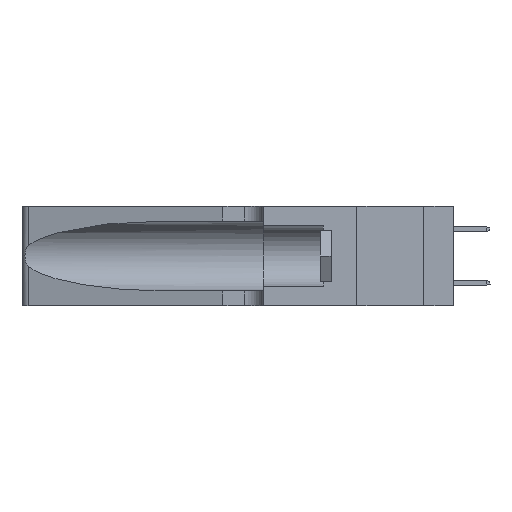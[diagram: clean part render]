
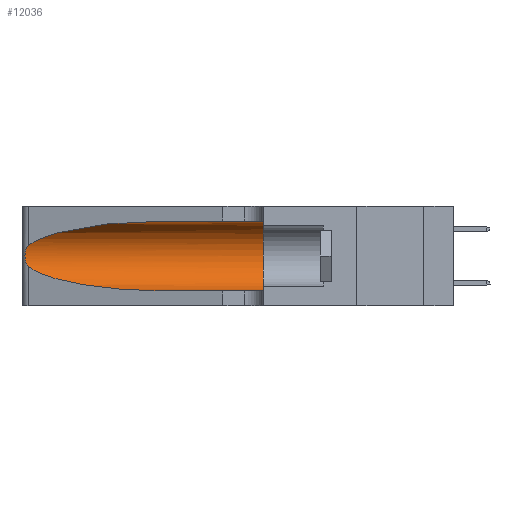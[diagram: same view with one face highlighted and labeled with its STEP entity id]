
A CAD part, left-side view. The second image highlights one B-rep face of the part: STEP entity #12036.
In plain terms, the highlighted cylindrical face has radius 3.308 mm (diameter 6.617 mm), a partial arc.
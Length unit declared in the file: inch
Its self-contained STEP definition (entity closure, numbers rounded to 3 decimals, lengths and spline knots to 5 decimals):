
#126 = CARTESIAN_POINT ( 'NONE',  ( 0.1305, 0.72297, 0.31525 ) ) ;
#168 = EDGE_CURVE ( 'NONE', #28024, #10101, #373, .T. ) ;
#373 = LINE ( 'NONE', #2477, #8485 ) ;
#961 = CARTESIAN_POINT ( 'NONE',  ( 0.1305, 0.72297, 0.31525 ) ) ;
#2454 = CARTESIAN_POINT ( 'NONE',  ( 0.1305, 0.35, 0.31525 ) ) ;
#2477 = CARTESIAN_POINT ( 'NONE',  ( 0.1305, 1.61858, 0.31525 ) ) ;
#3458 = EDGE_CURVE ( 'NONE', #17336, #17997, #14928, .T. ) ;
#3808 = CARTESIAN_POINT ( 'NONE',  ( 0.25856, 1.23593, 0.16098 ) ) ;
#3963 = CARTESIAN_POINT ( 'NONE',  ( 0.25789, 1.23486, 0.15765 ) ) ;
#4413 = LINE ( 'NONE', #13510, #17447 ) ;
#4511 = CARTESIAN_POINT ( 'NONE',  ( 0.1305, 0.72297, 0.05475 ) ) ;
#4795 = EDGE_CURVE ( 'NONE', #27685, #5377, #4413, .T. ) ;
#5363 = CARTESIAN_POINT ( 'NONE',  ( 0.2373, 1.15595, 0.08982 ) ) ;
#5377 = VERTEX_POINT ( 'NONE', #28081 ) ;
#7649 = AXIS2_PLACEMENT_3D ( 'NONE', #28971, #24512, #13146 ) ;
#8152 = AXIS2_PLACEMENT_3D ( 'NONE', #21940, #28342, #19832 ) ;
#8485 = VECTOR ( 'NONE', #12420, 39.37008 ) ;
#10094 = CARTESIAN_POINT ( 'NONE',  ( 0.18966, 0.96281, 0.31525 ) ) ;
#10101 = VERTEX_POINT ( 'NONE', #2454 ) ;
#10274 = CARTESIAN_POINT ( 'NONE',  ( 0.25487, 1.22718, 0.14631 ) ) ;
#10445 = CYLINDRICAL_SURFACE ( 'NONE', #8152, 0.13025 ) ;
#10976 = CARTESIAN_POINT ( 'NONE',  ( 0.25854, 1.2359, 0.20912 ) ) ;
#11126 = CARTESIAN_POINT ( 'NONE',  ( 0.25555, 1.22994, 0.2215 ) ) ;
#11644 = EDGE_CURVE ( 'NONE', #10101, #5377, #20506, .T. ) ;
#12036 = ADVANCED_FACE ( 'NONE', ( #12517 ), #10445, .F. ) ;
#12420 = DIRECTION ( 'NONE',  ( 0., -1., 0. ) ) ;
#12517 = FACE_OUTER_BOUND ( 'NONE', #25719, .T. ) ;
#12912 = CARTESIAN_POINT ( 'NONE',  ( 0.25555, 1.22993, 0.14849 ) ) ;
#13146 = DIRECTION ( 'NONE',  ( 0., 0., 1. ) ) ;
#13510 = CARTESIAN_POINT ( 'NONE',  ( 0.1305, 1.61858, 0.05475 ) ) ;
#13924 = ORIENTED_EDGE ( 'NONE', *, *, #28199, .T. ) ;
#14928 = B_SPLINE_CURVE_WITH_KNOTS ( 'NONE', 3,
 ( #19634, #11126, #27082, #26797, #10976, #26934, #26640, #20226, #24425, #3808, #3963, #19775, #12912, #29319 ),
 .UNSPECIFIED., .F., .F.,
 ( 4, 2, 2, 2, 2, 2, 4 ),
 ( 0., 0.00027, 0.00053, 0.00107, 0.0016, 0.00187, 0.00214 ),
 .UNSPECIFIED. ) ;
#16085 = ORIENTED_EDGE ( 'NONE', *, *, #168, .F. ) ;
#16308 = ORIENTED_EDGE ( 'NONE', *, *, #4795, .T. ) ;
#16701 = CARTESIAN_POINT ( 'NONE',  ( 0.1305, 0.72297, 0.05475 ) ) ;
#16946 = CARTESIAN_POINT ( 'NONE',  ( 0.2373, 1.15595, 0.28018 ) ) ;
#17028 =( BOUNDED_CURVE ( )  B_SPLINE_CURVE ( 3, ( #961, #10094, #16946, #21593 ),
 .UNSPECIFIED., .F., .T. ) 
 B_SPLINE_CURVE_WITH_KNOTS ( ( 4, 4 ),
 ( 1.5708, 2.84003 ),
 .UNSPECIFIED. ) 
 CURVE ( )  GEOMETRIC_REPRESENTATION_ITEM ( )  RATIONAL_B_SPLINE_CURVE ( ( 1., 0.87, 0.87, 1. ) ) 
 REPRESENTATION_ITEM ( '' )  );
#17336 = VERTEX_POINT ( 'NONE', #27878 ) ;
#17382 = CARTESIAN_POINT ( 'NONE',  ( 0.25487, 1.22718, 0.14631 ) ) ;
#17447 = VECTOR ( 'NONE', #20089, 39.37008 ) ;
#17997 = VERTEX_POINT ( 'NONE', #17382 ) ;
#19634 = CARTESIAN_POINT ( 'NONE',  ( 0.25487, 1.22718, 0.22369 ) ) ;
#19775 = CARTESIAN_POINT ( 'NONE',  ( 0.25639, 1.23186, 0.15144 ) ) ;
#19832 = DIRECTION ( 'NONE',  ( 0., 0., -1. ) ) ;
#20089 = DIRECTION ( 'NONE',  ( 0., -1., 0. ) ) ;
#20226 = CARTESIAN_POINT ( 'NONE',  ( 0.26075, 1.23896, 0.178 ) ) ;
#20506 = CIRCLE ( 'NONE', #7649, 0.13025 ) ;
#21593 = CARTESIAN_POINT ( 'NONE',  ( 0.25487, 1.22718, 0.22369 ) ) ;
#21721 = EDGE_CURVE ( 'NONE', #28024, #17336, #17028, .T. ) ;
#21940 = CARTESIAN_POINT ( 'NONE',  ( 0.1305, 1.61858, 0.185 ) ) ;
#24425 = CARTESIAN_POINT ( 'NONE',  ( 0.26017, 1.23833, 0.17102 ) ) ;
#24512 = DIRECTION ( 'NONE',  ( 0., 1., 0. ) ) ;
#24735 = ORIENTED_EDGE ( 'NONE', *, *, #11644, .F. ) ;
#25719 = EDGE_LOOP ( 'NONE', ( #25825, #28984, #13924, #16308, #24735, #16085 ) ) ;
#25808 = CARTESIAN_POINT ( 'NONE',  ( 0.18966, 0.96281, 0.05475 ) ) ;
#25825 = ORIENTED_EDGE ( 'NONE', *, *, #21721, .T. ) ;
#26363 =( BOUNDED_CURVE ( )  B_SPLINE_CURVE ( 3, ( #10274, #5363, #25808, #16701 ),
 .UNSPECIFIED., .F., .T. ) 
 B_SPLINE_CURVE_WITH_KNOTS ( ( 4, 4 ),
 ( 3.44316, 4.71239 ),
 .UNSPECIFIED. ) 
 CURVE ( )  GEOMETRIC_REPRESENTATION_ITEM ( )  RATIONAL_B_SPLINE_CURVE ( ( 1., 0.87, 0.87, 1. ) ) 
 REPRESENTATION_ITEM ( '' )  );
#26640 = CARTESIAN_POINT ( 'NONE',  ( 0.26075, 1.23896, 0.19203 ) ) ;
#26797 = CARTESIAN_POINT ( 'NONE',  ( 0.25787, 1.23484, 0.2124 ) ) ;
#26934 = CARTESIAN_POINT ( 'NONE',  ( 0.26018, 1.23835, 0.19895 ) ) ;
#27082 = CARTESIAN_POINT ( 'NONE',  ( 0.25639, 1.23184, 0.21858 ) ) ;
#27685 = VERTEX_POINT ( 'NONE', #4511 ) ;
#27878 = CARTESIAN_POINT ( 'NONE',  ( 0.25487, 1.22718, 0.22369 ) ) ;
#28024 = VERTEX_POINT ( 'NONE', #126 ) ;
#28081 = CARTESIAN_POINT ( 'NONE',  ( 0.1305, 0.35, 0.05475 ) ) ;
#28199 = EDGE_CURVE ( 'NONE', #17997, #27685, #26363, .T. ) ;
#28342 = DIRECTION ( 'NONE',  ( 0., -1., 0. ) ) ;
#28971 = CARTESIAN_POINT ( 'NONE',  ( 0.1305, 0.35, 0.185 ) ) ;
#28984 = ORIENTED_EDGE ( 'NONE', *, *, #3458, .T. ) ;
#29319 = CARTESIAN_POINT ( 'NONE',  ( 0.25487, 1.22718, 0.14631 ) ) ;
